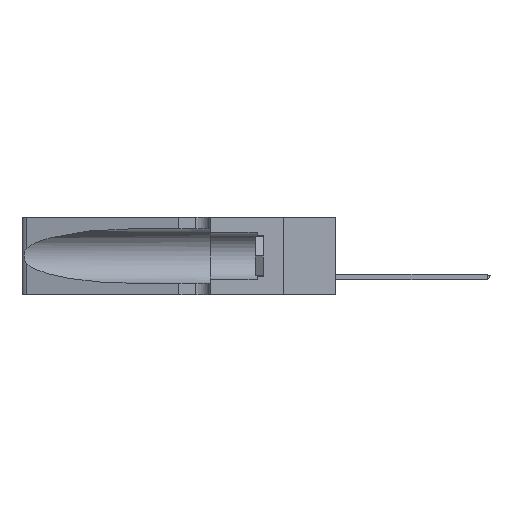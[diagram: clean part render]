
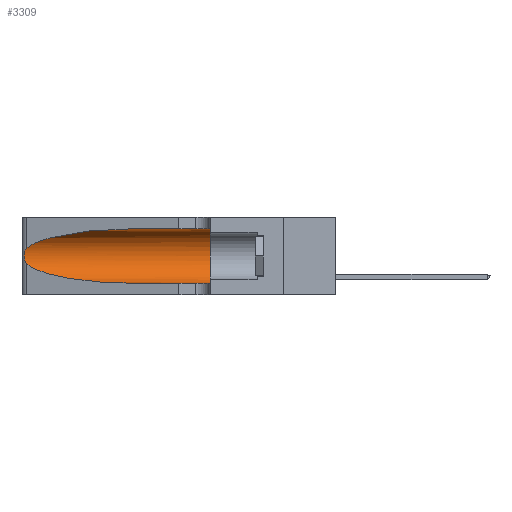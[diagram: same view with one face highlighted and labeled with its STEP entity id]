
A CAD part, left-side view. The second image highlights one B-rep face of the part: STEP entity #3309.
In plain terms, the highlighted cylindrical face has radius 3.308 mm (diameter 6.617 mm), a partial arc.
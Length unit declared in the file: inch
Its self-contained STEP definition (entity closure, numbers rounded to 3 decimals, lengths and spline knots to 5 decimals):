
#962 = ORIENTED_EDGE ( 'NONE', *, *, #14997, .T. ) ;
#1627 = CARTESIAN_POINT ( 'NONE',  ( 0.26075, 1.23896, 0.19203 ) ) ;
#1962 = LINE ( 'NONE', #33978, #3869 ) ;
#2351 = CARTESIAN_POINT ( 'NONE',  ( 0.25487, 1.22718, 0.22369 ) ) ;
#3309 = ADVANCED_FACE ( 'NONE', ( #14984 ), #18628, .F. ) ;
#3869 = VECTOR ( 'NONE', #8203, 39.37008 ) ;
#5934 = EDGE_CURVE ( 'NONE', #46880, #16757, #33939, .T. ) ;
#6380 = CARTESIAN_POINT ( 'NONE',  ( 0.25555, 1.22994, 0.2215 ) ) ;
#8203 = DIRECTION ( 'NONE',  ( 0., -1., 0. ) ) ;
#9688 = DIRECTION ( 'NONE',  ( 0., 0., 1. ) ) ;
#9907 = CARTESIAN_POINT ( 'NONE',  ( 0.1305, 0.35, 0.05475 ) ) ;
#10048 = EDGE_CURVE ( 'NONE', #27715, #27506, #47097, .T. ) ;
#10356 = CARTESIAN_POINT ( 'NONE',  ( 0.25639, 1.23184, 0.21858 ) ) ;
#10679 =( BOUNDED_CURVE ( )  B_SPLINE_CURVE ( 3, ( #27658, #40963, #16865, #12542 ),
 .UNSPECIFIED., .F., .T. ) 
 B_SPLINE_CURVE_WITH_KNOTS ( ( 4, 4 ),
 ( 3.44316, 4.71239 ),
 .UNSPECIFIED. ) 
 CURVE ( )  GEOMETRIC_REPRESENTATION_ITEM ( )  RATIONAL_B_SPLINE_CURVE ( ( 1., 0.87, 0.87, 1. ) ) 
 REPRESENTATION_ITEM ( '' )  );
#11690 = ORIENTED_EDGE ( 'NONE', *, *, #10048, .T. ) ;
#12542 = CARTESIAN_POINT ( 'NONE',  ( 0.1305, 0.72297, 0.05475 ) ) ;
#12697 = VECTOR ( 'NONE', #29966, 39.37008 ) ;
#13565 = DIRECTION ( 'NONE',  ( 0., 1., 0. ) ) ;
#14044 = CARTESIAN_POINT ( 'NONE',  ( 0.26017, 1.23833, 0.17102 ) ) ;
#14383 = CARTESIAN_POINT ( 'NONE',  ( 0.26018, 1.23835, 0.19895 ) ) ;
#14511 = B_SPLINE_CURVE_WITH_KNOTS ( 'NONE', 3,
 ( #2351, #6380, #10356, #29790, #38259, #14383, #1627, #29606, #14044, #41938, #41761, #18359, #21417, #21588 ),
 .UNSPECIFIED., .F., .F.,
 ( 4, 2, 2, 2, 2, 2, 4 ),
 ( 0., 0.00027, 0.00053, 0.00107, 0.0016, 0.00187, 0.00214 ),
 .UNSPECIFIED. ) ;
#14984 = FACE_OUTER_BOUND ( 'NONE', #40342, .T. ) ;
#14997 = EDGE_CURVE ( 'NONE', #16757, #30615, #14511, .T. ) ;
#15698 = CARTESIAN_POINT ( 'NONE',  ( 0.1305, 1.61858, 0.05475 ) ) ;
#16757 = VERTEX_POINT ( 'NONE', #38224 ) ;
#16865 = CARTESIAN_POINT ( 'NONE',  ( 0.18966, 0.96281, 0.05475 ) ) ;
#17024 = ORIENTED_EDGE ( 'NONE', *, *, #42081, .T. ) ;
#17987 = CARTESIAN_POINT ( 'NONE',  ( 0.25487, 1.22718, 0.14631 ) ) ;
#18147 = EDGE_CURVE ( 'NONE', #27014, #27506, #34805, .T. ) ;
#18359 = CARTESIAN_POINT ( 'NONE',  ( 0.25639, 1.23186, 0.15144 ) ) ;
#18628 = CYLINDRICAL_SURFACE ( 'NONE', #32164, 0.13025 ) ;
#20928 = ORIENTED_EDGE ( 'NONE', *, *, #18147, .F. ) ;
#21417 = CARTESIAN_POINT ( 'NONE',  ( 0.25555, 1.22993, 0.14849 ) ) ;
#21569 = CARTESIAN_POINT ( 'NONE',  ( 0.1305, 0.35, 0.31525 ) ) ;
#21588 = CARTESIAN_POINT ( 'NONE',  ( 0.25487, 1.22718, 0.14631 ) ) ;
#23025 = ORIENTED_EDGE ( 'NONE', *, *, #44176, .F. ) ;
#24770 = CARTESIAN_POINT ( 'NONE',  ( 0.25487, 1.22718, 0.22369 ) ) ;
#25459 = CARTESIAN_POINT ( 'NONE',  ( 0.1305, 0.35, 0.185 ) ) ;
#27014 = VERTEX_POINT ( 'NONE', #21569 ) ;
#27094 = CARTESIAN_POINT ( 'NONE',  ( 0.1305, 1.61858, 0.185 ) ) ;
#27267 = DIRECTION ( 'NONE',  ( 0., 0., -1. ) ) ;
#27506 = VERTEX_POINT ( 'NONE', #9907 ) ;
#27553 = AXIS2_PLACEMENT_3D ( 'NONE', #25459, #13565, #9688 ) ;
#27658 = CARTESIAN_POINT ( 'NONE',  ( 0.25487, 1.22718, 0.14631 ) ) ;
#27715 = VERTEX_POINT ( 'NONE', #29744 ) ;
#29606 = CARTESIAN_POINT ( 'NONE',  ( 0.26075, 1.23896, 0.178 ) ) ;
#29744 = CARTESIAN_POINT ( 'NONE',  ( 0.1305, 0.72297, 0.05475 ) ) ;
#29790 = CARTESIAN_POINT ( 'NONE',  ( 0.25787, 1.23484, 0.2124 ) ) ;
#29966 = DIRECTION ( 'NONE',  ( 0., -1., 0. ) ) ;
#30615 = VERTEX_POINT ( 'NONE', #17987 ) ;
#32164 = AXIS2_PLACEMENT_3D ( 'NONE', #27094, #35369, #27267 ) ;
#33882 = CARTESIAN_POINT ( 'NONE',  ( 0.1305, 0.72297, 0.31525 ) ) ;
#33939 =( BOUNDED_CURVE ( )  B_SPLINE_CURVE ( 3, ( #41662, #37445, #37620, #24770 ),
 .UNSPECIFIED., .F., .T. ) 
 B_SPLINE_CURVE_WITH_KNOTS ( ( 4, 4 ),
 ( 1.5708, 2.84003 ),
 .UNSPECIFIED. ) 
 CURVE ( )  GEOMETRIC_REPRESENTATION_ITEM ( )  RATIONAL_B_SPLINE_CURVE ( ( 1., 0.87, 0.87, 1. ) ) 
 REPRESENTATION_ITEM ( '' )  );
#33978 = CARTESIAN_POINT ( 'NONE',  ( 0.1305, 1.61858, 0.31525 ) ) ;
#34805 = CIRCLE ( 'NONE', #27553, 0.13025 ) ;
#35369 = DIRECTION ( 'NONE',  ( 0., -1., 0. ) ) ;
#37445 = CARTESIAN_POINT ( 'NONE',  ( 0.18966, 0.96281, 0.31525 ) ) ;
#37620 = CARTESIAN_POINT ( 'NONE',  ( 0.2373, 1.15595, 0.28018 ) ) ;
#38224 = CARTESIAN_POINT ( 'NONE',  ( 0.25487, 1.22718, 0.22369 ) ) ;
#38259 = CARTESIAN_POINT ( 'NONE',  ( 0.25854, 1.2359, 0.20912 ) ) ;
#40342 = EDGE_LOOP ( 'NONE', ( #49029, #962, #17024, #11690, #20928, #23025 ) ) ;
#40963 = CARTESIAN_POINT ( 'NONE',  ( 0.2373, 1.15595, 0.08982 ) ) ;
#41662 = CARTESIAN_POINT ( 'NONE',  ( 0.1305, 0.72297, 0.31525 ) ) ;
#41761 = CARTESIAN_POINT ( 'NONE',  ( 0.25789, 1.23486, 0.15765 ) ) ;
#41938 = CARTESIAN_POINT ( 'NONE',  ( 0.25856, 1.23593, 0.16098 ) ) ;
#42081 = EDGE_CURVE ( 'NONE', #30615, #27715, #10679, .T. ) ;
#44176 = EDGE_CURVE ( 'NONE', #46880, #27014, #1962, .T. ) ;
#46880 = VERTEX_POINT ( 'NONE', #33882 ) ;
#47097 = LINE ( 'NONE', #15698, #12697 ) ;
#49029 = ORIENTED_EDGE ( 'NONE', *, *, #5934, .T. ) ;
